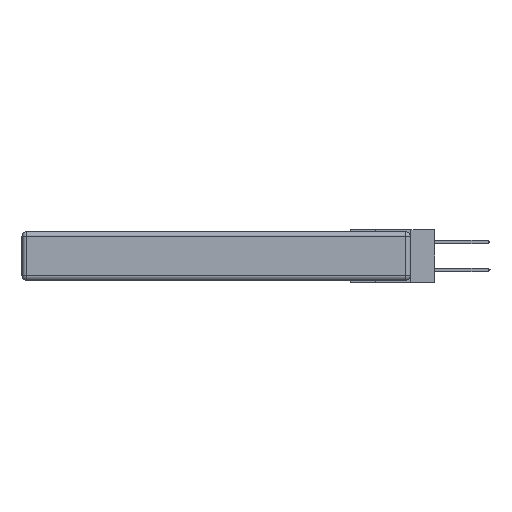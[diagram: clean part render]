
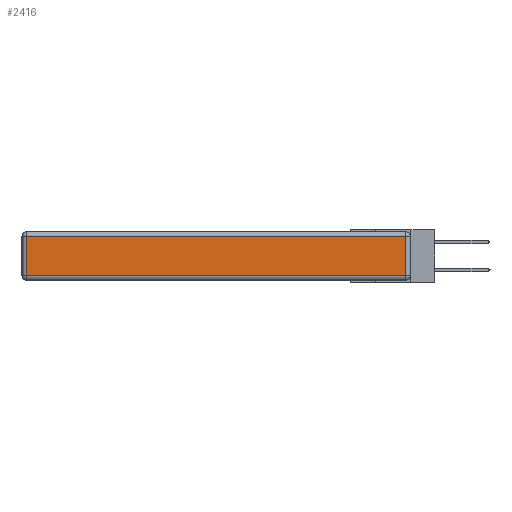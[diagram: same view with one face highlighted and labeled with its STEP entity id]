
A CAD part, left-side view. The second image highlights one B-rep face of the part: STEP entity #2416.
In plain terms, the highlighted planar face has unit normal (-1, 0, 0).
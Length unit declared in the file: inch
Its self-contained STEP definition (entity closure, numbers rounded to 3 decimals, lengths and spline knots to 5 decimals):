
#256 = CARTESIAN_POINT ( 'NONE',  ( 0., 2.75, -0.03 ) ) ;
#1362 = VECTOR ( 'NONE', #17612, 39.37008 ) ;
#2155 = VERTEX_POINT ( 'NONE', #7701 ) ;
#2416 = ADVANCED_FACE ( 'NONE', ( #18809 ), #17370, .T. ) ;
#2923 = VERTEX_POINT ( 'NONE', #10085 ) ;
#3233 = CARTESIAN_POINT ( 'NONE',  ( 0., 0., -0.343 ) ) ;
#3602 = CARTESIAN_POINT ( 'NONE',  ( 0., 0.03, -0.343 ) ) ;
#4542 = ORIENTED_EDGE ( 'NONE', *, *, #18944, .T. ) ;
#5139 = ORIENTED_EDGE ( 'NONE', *, *, #14289, .T. ) ;
#5436 = CARTESIAN_POINT ( 'NONE',  ( 0., 0., -0.313 ) ) ;
#5488 = LINE ( 'NONE', #3602, #1362 ) ;
#6528 = VERTEX_POINT ( 'NONE', #13482 ) ;
#6766 = VECTOR ( 'NONE', #14726, 39.37008 ) ;
#7701 = CARTESIAN_POINT ( 'NONE',  ( 0., 0.03, -0.03 ) ) ;
#8141 = DIRECTION ( 'NONE',  ( -1., 0., 0. ) ) ;
#8382 = DIRECTION ( 'NONE',  ( 0., 0., -1. ) ) ;
#9175 = LINE ( 'NONE', #13091, #11565 ) ;
#9242 = EDGE_CURVE ( 'NONE', #6528, #2155, #5488, .T. ) ;
#10085 = CARTESIAN_POINT ( 'NONE',  ( 0., 2.72, -0.03 ) ) ;
#10647 = LINE ( 'NONE', #256, #18298 ) ;
#11134 = DIRECTION ( 'NONE',  ( 0., 1., 0. ) ) ;
#11565 = VECTOR ( 'NONE', #8382, 39.37008 ) ;
#11822 = LINE ( 'NONE', #5436, #6766 ) ;
#12582 = EDGE_LOOP ( 'NONE', ( #19040, #18184, #5139, #4542 ) ) ;
#13091 = CARTESIAN_POINT ( 'NONE',  ( 0., 2.72, -0.343 ) ) ;
#13482 = CARTESIAN_POINT ( 'NONE',  ( 0., 0.03, -0.313 ) ) ;
#13908 = EDGE_CURVE ( 'NONE', #14496, #6528, #11822, .T. ) ;
#14289 = EDGE_CURVE ( 'NONE', #2155, #2923, #10647, .T. ) ;
#14496 = VERTEX_POINT ( 'NONE', #17665 ) ;
#14726 = DIRECTION ( 'NONE',  ( 0., -1., 0. ) ) ;
#15859 = AXIS2_PLACEMENT_3D ( 'NONE', #3233, #8141, #17173 ) ;
#17173 = DIRECTION ( 'NONE',  ( 0., 0., 1. ) ) ;
#17370 = PLANE ( 'NONE',  #15859 ) ;
#17612 = DIRECTION ( 'NONE',  ( 0., 0., 1. ) ) ;
#17665 = CARTESIAN_POINT ( 'NONE',  ( 0., 2.72, -0.313 ) ) ;
#18184 = ORIENTED_EDGE ( 'NONE', *, *, #9242, .T. ) ;
#18298 = VECTOR ( 'NONE', #11134, 39.37008 ) ;
#18809 = FACE_OUTER_BOUND ( 'NONE', #12582, .T. ) ;
#18944 = EDGE_CURVE ( 'NONE', #2923, #14496, #9175, .T. ) ;
#19040 = ORIENTED_EDGE ( 'NONE', *, *, #13908, .T. ) ;
